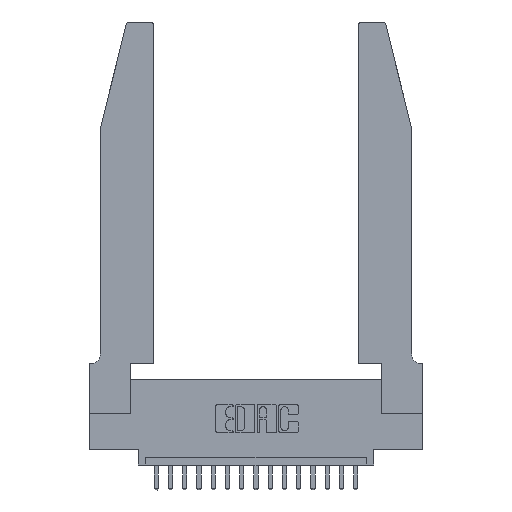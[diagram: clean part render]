
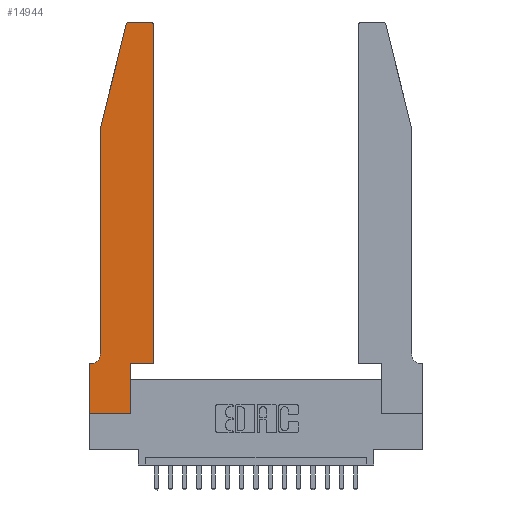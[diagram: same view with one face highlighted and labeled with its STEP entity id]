
A CAD part, top view. The second image highlights one B-rep face of the part: STEP entity #14944.
In plain terms, the highlighted planar face has unit normal (0, 0, 1).
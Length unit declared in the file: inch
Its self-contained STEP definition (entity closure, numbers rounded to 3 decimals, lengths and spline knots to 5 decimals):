
#298 = DIRECTION ( 'NONE',  ( 0., -1., 0. ) ) ;
#301 = DIRECTION ( 'NONE',  ( 0., -1., 0. ) ) ;
#522 = EDGE_CURVE ( 'NONE', #4526, #2161, #7939, .T. ) ;
#975 = EDGE_CURVE ( 'NONE', #6123, #8944, #17015, .T. ) ;
#1162 = VECTOR ( 'NONE', #13094, 39.37008 ) ;
#1248 = ORIENTED_EDGE ( 'NONE', *, *, #4328, .T. ) ;
#1430 = LINE ( 'NONE', #7587, #8655 ) ;
#1924 = EDGE_LOOP ( 'NONE', ( #4030, #10723, #16774, #13082, #16786, #12453, #5486, #3183, #8015, #1248, #2498, #11840 ) ) ;
#1947 = EDGE_CURVE ( 'NONE', #10122, #6123, #3569, .T. ) ;
#2005 = FACE_OUTER_BOUND ( 'NONE', #1924, .T. ) ;
#2161 = VERTEX_POINT ( 'NONE', #10744 ) ;
#2343 = CARTESIAN_POINT ( 'NONE',  ( 0.0055, 0.35, 0.37 ) ) ;
#2498 = ORIENTED_EDGE ( 'NONE', *, *, #11055, .T. ) ;
#3037 = DIRECTION ( 'NONE',  ( 1., 0., 0. ) ) ;
#3081 = CARTESIAN_POINT ( 'NONE',  ( 0.25487, 2.72718, 0.37 ) ) ;
#3090 = CARTESIAN_POINT ( 'NONE',  ( 0., 0.35, 0.37 ) ) ;
#3095 = CARTESIAN_POINT ( 'NONE',  ( 0., 0.35, 0.37 ) ) ;
#3183 = ORIENTED_EDGE ( 'NONE', *, *, #1947, .T. ) ;
#3242 = CIRCLE ( 'NONE', #5671, 0.03 ) ;
#3494 = DIRECTION ( 'NONE',  ( 0., 0., -1. ) ) ;
#3569 = LINE ( 'NONE', #9881, #19908 ) ;
#3702 = CARTESIAN_POINT ( 'NONE',  ( 0.0755, 0.42, 0.37 ) ) ;
#4030 = ORIENTED_EDGE ( 'NONE', *, *, #6806, .T. ) ;
#4109 = CARTESIAN_POINT ( 'NONE',  ( 0.0755, 2., 0.37 ) ) ;
#4328 = EDGE_CURVE ( 'NONE', #8944, #12009, #11886, .T. ) ;
#4420 = DIRECTION ( 'NONE',  ( 1., 0., 0. ) ) ;
#4526 = VERTEX_POINT ( 'NONE', #3081 ) ;
#4647 = CARTESIAN_POINT ( 'NONE',  ( 0.284, 2.72, 0.37 ) ) ;
#4671 = DIRECTION ( 'NONE',  ( -1., 0., 0. ) ) ;
#4942 = LINE ( 'NONE', #14673, #7858 ) ;
#5339 = CARTESIAN_POINT ( 'NONE',  ( 0.4505, 2.72, 0.37 ) ) ;
#5460 = DIRECTION ( 'NONE',  ( -1., 0., 0. ) ) ;
#5486 = ORIENTED_EDGE ( 'NONE', *, *, #12041, .T. ) ;
#5671 = AXIS2_PLACEMENT_3D ( 'NONE', #13624, #10443, #4420 ) ;
#6023 = DIRECTION ( 'NONE',  ( 1., 0., 0. ) ) ;
#6123 = VERTEX_POINT ( 'NONE', #12098 ) ;
#6465 = LINE ( 'NONE', #15379, #6921 ) ;
#6806 = EDGE_CURVE ( 'NONE', #19825, #19244, #4942, .T. ) ;
#6921 = VECTOR ( 'NONE', #298, 39.37008 ) ;
#7204 = LINE ( 'NONE', #19021, #17769 ) ;
#7584 = VERTEX_POINT ( 'NONE', #3090 ) ;
#7587 = CARTESIAN_POINT ( 'NONE',  ( 0.0755, 0.35, 0.37 ) ) ;
#7632 = AXIS2_PLACEMENT_3D ( 'NONE', #9764, #3494, #12688 ) ;
#7858 = VECTOR ( 'NONE', #5460, 39.37008 ) ;
#7875 = DIRECTION ( 'NONE',  ( 1., 0., 0. ) ) ;
#7939 = LINE ( 'NONE', #4109, #1162 ) ;
#8015 = ORIENTED_EDGE ( 'NONE', *, *, #975, .T. ) ;
#8083 = CARTESIAN_POINT ( 'NONE',  ( 0.0755, 2., 0.37 ) ) ;
#8322 = CARTESIAN_POINT ( 'NONE',  ( 0.4205, 2.75, 0.37 ) ) ;
#8655 = VECTOR ( 'NONE', #4671, 39.37008 ) ;
#8743 = VERTEX_POINT ( 'NONE', #3702 ) ;
#8777 = AXIS2_PLACEMENT_3D ( 'NONE', #3095, #14094, #7875 ) ;
#8905 = VECTOR ( 'NONE', #301, 39.37008 ) ;
#8944 = VERTEX_POINT ( 'NONE', #10103 ) ;
#9368 = CARTESIAN_POINT ( 'NONE',  ( 0.4505, 0.35, 0.37 ) ) ;
#9764 = CARTESIAN_POINT ( 'NONE',  ( 0.0055, 0.42, 0.37 ) ) ;
#9833 = EDGE_CURVE ( 'NONE', #19244, #4526, #9880, .T. ) ;
#9880 = CIRCLE ( 'NONE', #18092, 0.03 ) ;
#9881 = CARTESIAN_POINT ( 'NONE',  ( 0., 0., 0.37 ) ) ;
#10103 = CARTESIAN_POINT ( 'NONE',  ( 0.2865, 0.35, 0.37 ) ) ;
#10120 = EDGE_CURVE ( 'NONE', #2161, #8743, #14649, .T. ) ;
#10122 = VERTEX_POINT ( 'NONE', #14238 ) ;
#10196 = VECTOR ( 'NONE', #3037, 39.37008 ) ;
#10443 = DIRECTION ( 'NONE',  ( 0., 0., 1. ) ) ;
#10723 = ORIENTED_EDGE ( 'NONE', *, *, #9833, .T. ) ;
#10744 = CARTESIAN_POINT ( 'NONE',  ( 0.0755, 2., 0.37 ) ) ;
#10920 = CARTESIAN_POINT ( 'NONE',  ( 0.4505, 0.35, 0.37 ) ) ;
#11055 = EDGE_CURVE ( 'NONE', #12009, #17696, #7204, .T. ) ;
#11062 = EDGE_CURVE ( 'NONE', #14468, #7584, #1430, .T. ) ;
#11840 = ORIENTED_EDGE ( 'NONE', *, *, #14808, .T. ) ;
#11886 = LINE ( 'NONE', #10920, #10196 ) ;
#12009 = VERTEX_POINT ( 'NONE', #9368 ) ;
#12041 = EDGE_CURVE ( 'NONE', #7584, #10122, #6465, .T. ) ;
#12098 = CARTESIAN_POINT ( 'NONE',  ( 0.2865, 0., 0.37 ) ) ;
#12259 = DIRECTION ( 'NONE',  ( 0., 0., 1. ) ) ;
#12453 = ORIENTED_EDGE ( 'NONE', *, *, #11062, .T. ) ;
#12602 = CIRCLE ( 'NONE', #7632, 0.07 ) ;
#12688 = DIRECTION ( 'NONE',  ( -1., 0., 0. ) ) ;
#13082 = ORIENTED_EDGE ( 'NONE', *, *, #10120, .T. ) ;
#13094 = DIRECTION ( 'NONE',  ( -0.239, -0.971, 0. ) ) ;
#13188 = DIRECTION ( 'NONE',  ( 1., 0., 0. ) ) ;
#13624 = CARTESIAN_POINT ( 'NONE',  ( 0.4205, 2.72, 0.37 ) ) ;
#14094 = DIRECTION ( 'NONE',  ( 0., 0., 1. ) ) ;
#14238 = CARTESIAN_POINT ( 'NONE',  ( 0., 0., 0.37 ) ) ;
#14468 = VERTEX_POINT ( 'NONE', #2343 ) ;
#14570 = CARTESIAN_POINT ( 'NONE',  ( 0.284, 2.75, 0.37 ) ) ;
#14649 = LINE ( 'NONE', #8083, #8905 ) ;
#14673 = CARTESIAN_POINT ( 'NONE',  ( 0.2605, 2.75, 0.37 ) ) ;
#14808 = EDGE_CURVE ( 'NONE', #17696, #19825, #3242, .T. ) ;
#14944 = ADVANCED_FACE ( 'NONE', ( #2005 ), #16967, .T. ) ;
#15064 = EDGE_CURVE ( 'NONE', #8743, #14468, #12602, .T. ) ;
#15379 = CARTESIAN_POINT ( 'NONE',  ( 0., 0., 0.37 ) ) ;
#16082 = DIRECTION ( 'NONE',  ( 0., 1., 0. ) ) ;
#16774 = ORIENTED_EDGE ( 'NONE', *, *, #522, .T. ) ;
#16786 = ORIENTED_EDGE ( 'NONE', *, *, #15064, .T. ) ;
#16855 = CARTESIAN_POINT ( 'NONE',  ( 0.2865, 0.35, 0.37 ) ) ;
#16967 = PLANE ( 'NONE',  #8777 ) ;
#17015 = LINE ( 'NONE', #16855, #19441 ) ;
#17696 = VERTEX_POINT ( 'NONE', #5339 ) ;
#17769 = VECTOR ( 'NONE', #16082, 39.37008 ) ;
#18092 = AXIS2_PLACEMENT_3D ( 'NONE', #4647, #12259, #6023 ) ;
#18375 = DIRECTION ( 'NONE',  ( 0., 1., 0. ) ) ;
#19021 = CARTESIAN_POINT ( 'NONE',  ( 0.4505, 0.35, 0.37 ) ) ;
#19244 = VERTEX_POINT ( 'NONE', #14570 ) ;
#19441 = VECTOR ( 'NONE', #18375, 39.37008 ) ;
#19825 = VERTEX_POINT ( 'NONE', #8322 ) ;
#19908 = VECTOR ( 'NONE', #13188, 39.37008 ) ;
